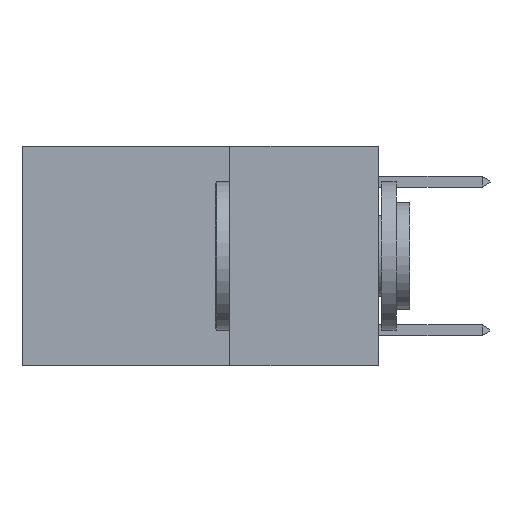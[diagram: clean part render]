
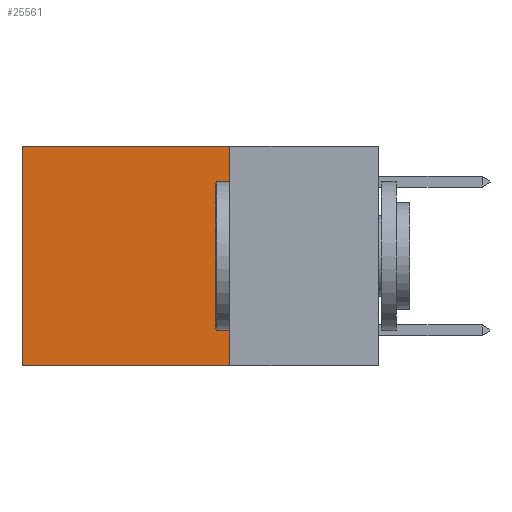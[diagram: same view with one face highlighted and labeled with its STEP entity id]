
A CAD part, left-side view. The second image highlights one B-rep face of the part: STEP entity #25561.
In plain terms, the highlighted planar face has unit normal (-1, 0, 0).
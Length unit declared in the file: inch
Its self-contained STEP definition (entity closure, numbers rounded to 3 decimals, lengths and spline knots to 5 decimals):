
#439 = DIRECTION ( 'NONE',  ( 0., 0., -1. ) ) ;
#2428 = CARTESIAN_POINT ( 'NONE',  ( 0.2625, 0.6, 0. ) ) ;
#5230 = LINE ( 'NONE', #15066, #24115 ) ;
#6974 = VECTOR ( 'NONE', #27185, 39.37008 ) ;
#7127 = CARTESIAN_POINT ( 'NONE',  ( 0.2625, 0.25, -0.37 ) ) ;
#7735 = LINE ( 'NONE', #2428, #29801 ) ;
#9724 = CARTESIAN_POINT ( 'NONE',  ( 0.2625, 0.6, -0.37 ) ) ;
#10537 = VERTEX_POINT ( 'NONE', #24837 ) ;
#12055 = EDGE_CURVE ( 'NONE', #15884, #10537, #5230, .T. ) ;
#12232 = CARTESIAN_POINT ( 'NONE',  ( 0.2625, 0.25, 0. ) ) ;
#12404 = LINE ( 'NONE', #17391, #6974 ) ;
#13719 = EDGE_LOOP ( 'NONE', ( #25288, #16621, #28520, #30700 ) ) ;
#13879 = FACE_OUTER_BOUND ( 'NONE', #13719, .T. ) ;
#14028 = VERTEX_POINT ( 'NONE', #9724 ) ;
#15066 = CARTESIAN_POINT ( 'NONE',  ( 0.2625, 0.25, 0. ) ) ;
#15884 = VERTEX_POINT ( 'NONE', #12232 ) ;
#16621 = ORIENTED_EDGE ( 'NONE', *, *, #19329, .F. ) ;
#17391 = CARTESIAN_POINT ( 'NONE',  ( 0.2625, 0.25, -0.37 ) ) ;
#19321 = DIRECTION ( 'NONE',  ( 1., 0., 0. ) ) ;
#19329 = EDGE_CURVE ( 'NONE', #31161, #14028, #12404, .T. ) ;
#20401 = EDGE_CURVE ( 'NONE', #15884, #31161, #20527, .T. ) ;
#20527 = LINE ( 'NONE', #27763, #25009 ) ;
#21740 = PLANE ( 'NONE',  #22937 ) ;
#22296 = DIRECTION ( 'NONE',  ( 0., 1., 0. ) ) ;
#22937 = AXIS2_PLACEMENT_3D ( 'NONE', #31065, #19321, #29131 ) ;
#24115 = VECTOR ( 'NONE', #22296, 39.37008 ) ;
#24295 = EDGE_CURVE ( 'NONE', #10537, #14028, #7735, .T. ) ;
#24837 = CARTESIAN_POINT ( 'NONE',  ( 0.2625, 0.6, 0. ) ) ;
#25009 = VECTOR ( 'NONE', #439, 39.37008 ) ;
#25288 = ORIENTED_EDGE ( 'NONE', *, *, #24295, .T. ) ;
#25561 = ADVANCED_FACE ( 'NONE', ( #13879 ), #21740, .F. ) ;
#27185 = DIRECTION ( 'NONE',  ( 0., 1., 0. ) ) ;
#27763 = CARTESIAN_POINT ( 'NONE',  ( 0.2625, 0.25, 0. ) ) ;
#28520 = ORIENTED_EDGE ( 'NONE', *, *, #20401, .F. ) ;
#29131 = DIRECTION ( 'NONE',  ( 0., 0., -1. ) ) ;
#29780 = DIRECTION ( 'NONE',  ( 0., 0., -1. ) ) ;
#29801 = VECTOR ( 'NONE', #29780, 39.37008 ) ;
#30700 = ORIENTED_EDGE ( 'NONE', *, *, #12055, .T. ) ;
#31065 = CARTESIAN_POINT ( 'NONE',  ( 0.2625, 0.25, 0. ) ) ;
#31161 = VERTEX_POINT ( 'NONE', #7127 ) ;
